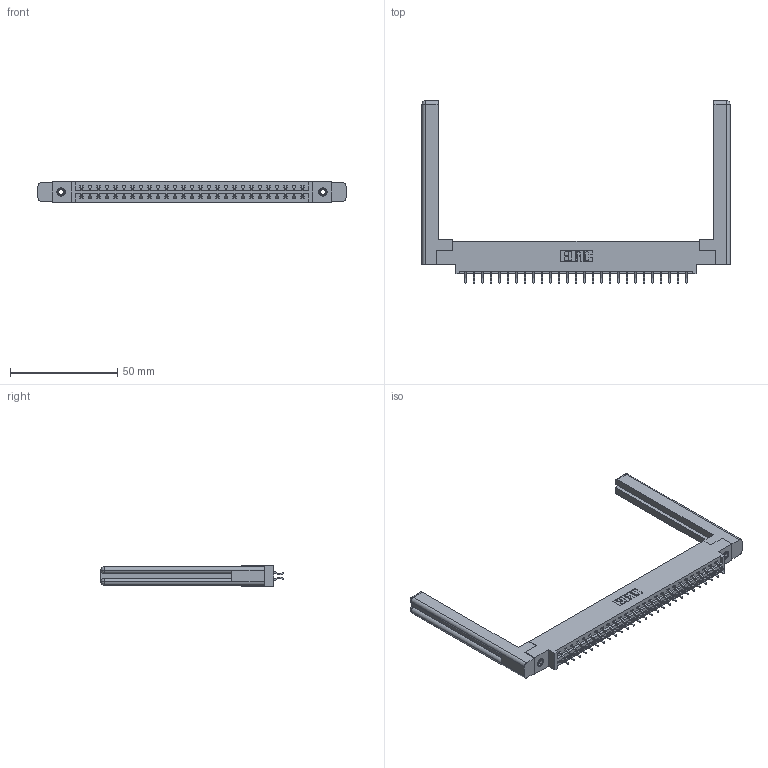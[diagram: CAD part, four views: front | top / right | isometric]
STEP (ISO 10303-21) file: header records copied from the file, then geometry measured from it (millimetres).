
FILE_DESCRIPTION (( 'STEP AP203' ), '1' );
FILE_NAME ('337-054-556-858.STEP', '2019-10-11T19:17:20', ( '' ), ( '' ), 'SwSTEP 2.0', 'SolidWorks 2016', '' );
FILE_SCHEMA (( 'CONFIG_CONTROL_DESIGN' ));
Length unit declared in the file: inch
Products named in the file (5): 345-292-001_556 Tail; 345-250-001_345-250-001-102; 337 Part_0.170 Offset - 0.156 Dia-TI; 337-054-556-858; 307-220-058
Assembly tree (59 placements, depth 2):
  337-054-556-858
    337 Part_0.170 Offset - 0.156 Dia-TI
    345-292-001_556 Tail  x54
    345-250-001_345-250-001-102  x2
    307-220-058  x2
Bounding box: 143.61 x 84.98 x 9.4 mm (x, y, z)
Volume: 21958 mm3; surface area: 21701 mm2
Topology: 59 solids, 59 shells, 3500 faces, 10343 edges, 6810 vertices
Faces by surface type: plane 2426, cylinder 1050, cone 12, torus 12
Entity records: 25860 total; most frequent: CARTESIAN_POINT 4393, ORIENTED_EDGE 4256, DIRECTION 3768, EDGE_CURVE 2128, VECTOR 1944, LINE 1944, VERTEX_POINT 1410, AXIS2_PLACEMENT_3D 912
